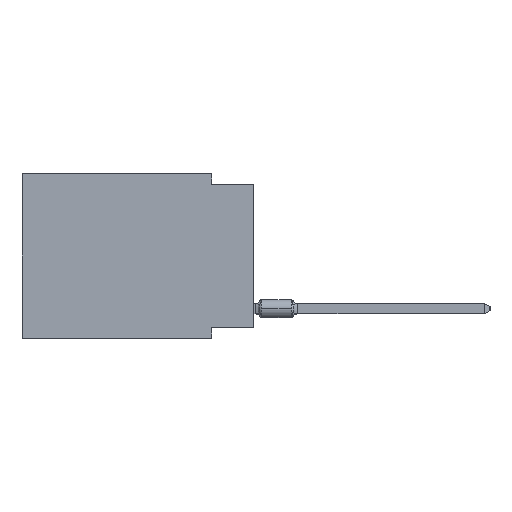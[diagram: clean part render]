
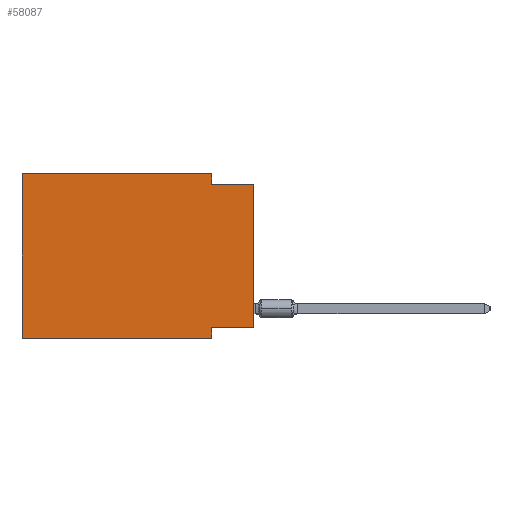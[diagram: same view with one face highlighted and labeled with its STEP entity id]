
A CAD part, left-side view. The second image highlights one B-rep face of the part: STEP entity #58087.
In plain terms, the highlighted planar face has unit normal (-1, 0, 0).
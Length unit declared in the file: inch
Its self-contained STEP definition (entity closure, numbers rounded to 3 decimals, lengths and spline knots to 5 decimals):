
#118 = CARTESIAN_POINT ( 'NONE',  ( 0., 0., -0.025 ) ) ;
#3850 = PLANE ( 'NONE',  #32590 ) ;
#6255 = DIRECTION ( 'NONE',  ( 0., 0., -1. ) ) ;
#7571 = CARTESIAN_POINT ( 'NONE',  ( 0., 0.1, 0. ) ) ;
#9199 = LINE ( 'NONE', #78267, #37600 ) ;
#9247 = EDGE_CURVE ( 'NONE', #61890, #70019, #9199, .T. ) ;
#9529 = LINE ( 'NONE', #50523, #87186 ) ;
#10655 = EDGE_CURVE ( 'NONE', #84220, #61890, #64202, .T. ) ;
#11622 = CARTESIAN_POINT ( 'NONE',  ( 0., 0.55, -0.39 ) ) ;
#13279 = EDGE_CURVE ( 'NONE', #53219, #26996, #31806, .T. ) ;
#13863 = EDGE_CURVE ( 'NONE', #70019, #22880, #68636, .T. ) ;
#15669 = LINE ( 'NONE', #118, #52819 ) ;
#17697 = FACE_OUTER_BOUND ( 'NONE', #21081, .T. ) ;
#18692 = ORIENTED_EDGE ( 'NONE', *, *, #13279, .T. ) ;
#19011 = CARTESIAN_POINT ( 'NONE',  ( 0., 0.1, -0.39 ) ) ;
#19308 = DIRECTION ( 'NONE',  ( 0., 0., 1. ) ) ;
#19893 = LINE ( 'NONE', #19011, #36343 ) ;
#20457 = CARTESIAN_POINT ( 'NONE',  ( 0., 0., -0.365 ) ) ;
#21081 = EDGE_LOOP ( 'NONE', ( #18692, #68915, #76128, #58816, #24759, #55268, #43168, #49184 ) ) ;
#22880 = VERTEX_POINT ( 'NONE', #58225 ) ;
#23003 = EDGE_CURVE ( 'NONE', #80972, #83313, #19893, .T. ) ;
#23499 = CARTESIAN_POINT ( 'NONE',  ( 0., 0.55, 0. ) ) ;
#24177 = CARTESIAN_POINT ( 'NONE',  ( 0., 0.1, 0. ) ) ;
#24759 = ORIENTED_EDGE ( 'NONE', *, *, #10655, .F. ) ;
#25347 = EDGE_CURVE ( 'NONE', #84220, #83313, #73550, .T. ) ;
#26238 = CARTESIAN_POINT ( 'NONE',  ( 0., 0., -0.025 ) ) ;
#26996 = VERTEX_POINT ( 'NONE', #26238 ) ;
#27755 = DIRECTION ( 'NONE',  ( 0., -1., 0. ) ) ;
#31800 = EDGE_CURVE ( 'NONE', #22880, #26996, #15669, .T. ) ;
#31806 = LINE ( 'NONE', #65661, #86264 ) ;
#32271 = VECTOR ( 'NONE', #6255, 39.37008 ) ;
#32590 = AXIS2_PLACEMENT_3D ( 'NONE', #23499, #59123, #78729 ) ;
#36343 = VECTOR ( 'NONE', #47950, 39.37008 ) ;
#37205 = CARTESIAN_POINT ( 'NONE',  ( 0., 0.1, -0.365 ) ) ;
#37600 = VECTOR ( 'NONE', #83197, 39.37008 ) ;
#37899 = CARTESIAN_POINT ( 'NONE',  ( 0., 0.55, 0. ) ) ;
#39226 = DIRECTION ( 'NONE',  ( 0., -1., 0. ) ) ;
#43168 = ORIENTED_EDGE ( 'NONE', *, *, #23003, .F. ) ;
#45039 = DIRECTION ( 'NONE',  ( 0., 0., 1. ) ) ;
#47950 = DIRECTION ( 'NONE',  ( 0., 0., -1. ) ) ;
#49184 = ORIENTED_EDGE ( 'NONE', *, *, #87594, .F. ) ;
#50523 = CARTESIAN_POINT ( 'NONE',  ( 0., 0., -0.365 ) ) ;
#52819 = VECTOR ( 'NONE', #27755, 39.37008 ) ;
#53219 = VERTEX_POINT ( 'NONE', #20457 ) ;
#55268 = ORIENTED_EDGE ( 'NONE', *, *, #25347, .T. ) ;
#58087 = ADVANCED_FACE ( 'NONE', ( #17697 ), #3850, .F. ) ;
#58225 = CARTESIAN_POINT ( 'NONE',  ( 0., 0.1, -0.025 ) ) ;
#58816 = ORIENTED_EDGE ( 'NONE', *, *, #9247, .F. ) ;
#59123 = DIRECTION ( 'NONE',  ( 1., 0., 0. ) ) ;
#61890 = VERTEX_POINT ( 'NONE', #62420 ) ;
#62420 = CARTESIAN_POINT ( 'NONE',  ( 0., 0.55, 0. ) ) ;
#64202 = LINE ( 'NONE', #37899, #75965 ) ;
#65091 = VECTOR ( 'NONE', #39226, 39.37008 ) ;
#65661 = CARTESIAN_POINT ( 'NONE',  ( 0., 0., 0. ) ) ;
#68636 = LINE ( 'NONE', #7571, #32271 ) ;
#68915 = ORIENTED_EDGE ( 'NONE', *, *, #31800, .F. ) ;
#70019 = VERTEX_POINT ( 'NONE', #24177 ) ;
#71463 = DIRECTION ( 'NONE',  ( 0., 1., 0. ) ) ;
#73550 = LINE ( 'NONE', #11622, #65091 ) ;
#74243 = CARTESIAN_POINT ( 'NONE',  ( 0., 0.1, -0.39 ) ) ;
#75965 = VECTOR ( 'NONE', #45039, 39.37008 ) ;
#76128 = ORIENTED_EDGE ( 'NONE', *, *, #13863, .F. ) ;
#78267 = CARTESIAN_POINT ( 'NONE',  ( 0., 0.55, 0. ) ) ;
#78729 = DIRECTION ( 'NONE',  ( 0., 0., -1. ) ) ;
#80972 = VERTEX_POINT ( 'NONE', #37205 ) ;
#83197 = DIRECTION ( 'NONE',  ( 0., -1., 0. ) ) ;
#83313 = VERTEX_POINT ( 'NONE', #74243 ) ;
#84220 = VERTEX_POINT ( 'NONE', #87702 ) ;
#86264 = VECTOR ( 'NONE', #19308, 39.37008 ) ;
#87186 = VECTOR ( 'NONE', #71463, 39.37008 ) ;
#87594 = EDGE_CURVE ( 'NONE', #53219, #80972, #9529, .T. ) ;
#87702 = CARTESIAN_POINT ( 'NONE',  ( 0., 0.55, -0.39 ) ) ;
